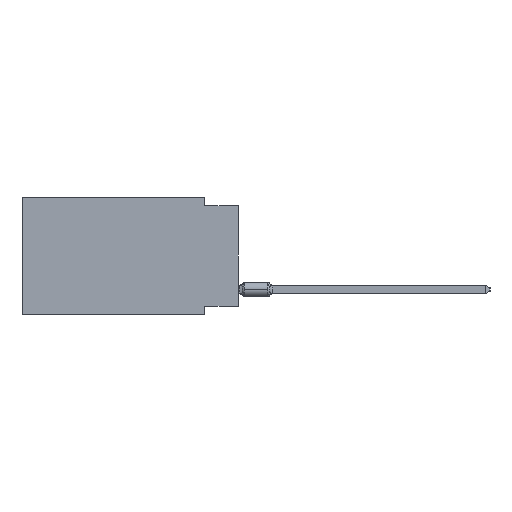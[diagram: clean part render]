
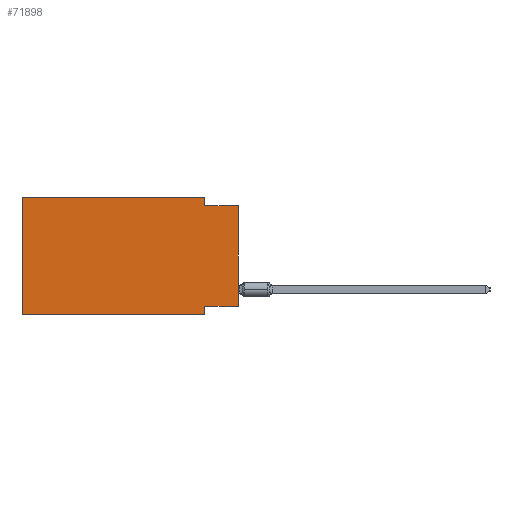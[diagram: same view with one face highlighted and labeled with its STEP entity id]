
A CAD part, left-side view. The second image highlights one B-rep face of the part: STEP entity #71898.
In plain terms, the highlighted planar face has unit normal (-1, 0, 0).
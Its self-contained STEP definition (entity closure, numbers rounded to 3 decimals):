
#1831 = VECTOR ( 'NONE', #77234, 1000. ) ;
#3227 = ORIENTED_EDGE ( 'NONE', *, *, #85287, .T. ) ;
#4537 = CARTESIAN_POINT ( 'NONE',  ( 0., 0., -0.635 ) ) ;
#5305 = LINE ( 'NONE', #25249, #21203 ) ;
#6075 = VECTOR ( 'NONE', #18033, 1000. ) ;
#7210 = ORIENTED_EDGE ( 'NONE', *, *, #81628, .F. ) ;
#7359 = ORIENTED_EDGE ( 'NONE', *, *, #38900, .F. ) ;
#11522 = DIRECTION ( 'NONE',  ( 0., 0., 1. ) ) ;
#11753 = ORIENTED_EDGE ( 'NONE', *, *, #20453, .F. ) ;
#14255 = CARTESIAN_POINT ( 'NONE',  ( 0., 0., -8.255 ) ) ;
#15845 = DIRECTION ( 'NONE',  ( 0., 0., 1. ) ) ;
#16922 = PLANE ( 'NONE',  #84972 ) ;
#17297 = LINE ( 'NONE', #45602, #70333 ) ;
#18033 = DIRECTION ( 'NONE',  ( 0., -1., 0. ) ) ;
#20453 = EDGE_CURVE ( 'NONE', #43171, #83432, #17297, .T. ) ;
#20618 = LINE ( 'NONE', #71031, #1831 ) ;
#21145 = CARTESIAN_POINT ( 'NONE',  ( 0., 16.383, -8.89 ) ) ;
#21203 = VECTOR ( 'NONE', #11522, 1000. ) ;
#21328 = VERTEX_POINT ( 'NONE', #14255 ) ;
#23291 = LINE ( 'NONE', #68447, #70757 ) ;
#25249 = CARTESIAN_POINT ( 'NONE',  ( 0., 0., 0. ) ) ;
#25520 = ORIENTED_EDGE ( 'NONE', *, *, #26877, .T. ) ;
#26877 = EDGE_CURVE ( 'NONE', #47099, #83432, #78660, .T. ) ;
#27640 = DIRECTION ( 'NONE',  ( 0., 0., -1. ) ) ;
#29930 = DIRECTION ( 'NONE',  ( 0., 1., 0. ) ) ;
#32141 = CARTESIAN_POINT ( 'NONE',  ( 0., 2.54, -8.255 ) ) ;
#35023 = VERTEX_POINT ( 'NONE', #84285 ) ;
#35749 = LINE ( 'NONE', #62773, #77316 ) ;
#38900 = EDGE_CURVE ( 'NONE', #47099, #35023, #35749, .T. ) ;
#39624 = LINE ( 'NONE', #46261, #44799 ) ;
#39806 = EDGE_LOOP ( 'NONE', ( #3227, #79651, #7210, #78888, #7359, #25520, #11753, #62754 ) ) ;
#39841 = LINE ( 'NONE', #53557, #54828 ) ;
#42591 = DIRECTION ( 'NONE',  ( 0., 0., -1. ) ) ;
#43171 = VERTEX_POINT ( 'NONE', #32141 ) ;
#44799 = VECTOR ( 'NONE', #27640, 1000. ) ;
#45602 = CARTESIAN_POINT ( 'NONE',  ( 0., 2.54, -8.89 ) ) ;
#46261 = CARTESIAN_POINT ( 'NONE',  ( 0., 2.54, 0. ) ) ;
#47099 = VERTEX_POINT ( 'NONE', #21145 ) ;
#47424 = VERTEX_POINT ( 'NONE', #52097 ) ;
#52097 = CARTESIAN_POINT ( 'NONE',  ( 0., 2.54, 0. ) ) ;
#53557 = CARTESIAN_POINT ( 'NONE',  ( 0., 0., -0.635 ) ) ;
#54108 = VERTEX_POINT ( 'NONE', #56656 ) ;
#54828 = VECTOR ( 'NONE', #81847, 1000. ) ;
#56656 = CARTESIAN_POINT ( 'NONE',  ( 0., 2.54, -0.635 ) ) ;
#61626 = CARTESIAN_POINT ( 'NONE',  ( 0., 2.54, -8.89 ) ) ;
#62754 = ORIENTED_EDGE ( 'NONE', *, *, #85864, .F. ) ;
#62773 = CARTESIAN_POINT ( 'NONE',  ( 0., 16.383, 0. ) ) ;
#68447 = CARTESIAN_POINT ( 'NONE',  ( 0., 0., -8.255 ) ) ;
#68719 = DIRECTION ( 'NONE',  ( 1., 0., 0. ) ) ;
#70333 = VECTOR ( 'NONE', #77931, 1000. ) ;
#70757 = VECTOR ( 'NONE', #29930, 1000. ) ;
#71031 = CARTESIAN_POINT ( 'NONE',  ( 0., 16.383, 0. ) ) ;
#71898 = ADVANCED_FACE ( 'NONE', ( #77120 ), #16922, .F. ) ;
#73950 = EDGE_CURVE ( 'NONE', #35023, #47424, #20618, .T. ) ;
#77120 = FACE_OUTER_BOUND ( 'NONE', #39806, .T. ) ;
#77234 = DIRECTION ( 'NONE',  ( 0., -1., 0. ) ) ;
#77316 = VECTOR ( 'NONE', #15845, 1000. ) ;
#77931 = DIRECTION ( 'NONE',  ( 0., 0., -1. ) ) ;
#78660 = LINE ( 'NONE', #85743, #6075 ) ;
#78888 = ORIENTED_EDGE ( 'NONE', *, *, #73950, .F. ) ;
#79546 = VERTEX_POINT ( 'NONE', #4537 ) ;
#79651 = ORIENTED_EDGE ( 'NONE', *, *, #82527, .F. ) ;
#81628 = EDGE_CURVE ( 'NONE', #47424, #54108, #39624, .T. ) ;
#81847 = DIRECTION ( 'NONE',  ( 0., -1., 0. ) ) ;
#82527 = EDGE_CURVE ( 'NONE', #54108, #79546, #39841, .T. ) ;
#83300 = CARTESIAN_POINT ( 'NONE',  ( 0., 16.383, 0. ) ) ;
#83432 = VERTEX_POINT ( 'NONE', #61626 ) ;
#84285 = CARTESIAN_POINT ( 'NONE',  ( 0., 16.383, 0. ) ) ;
#84972 = AXIS2_PLACEMENT_3D ( 'NONE', #83300, #68719, #42591 ) ;
#85287 = EDGE_CURVE ( 'NONE', #21328, #79546, #5305, .T. ) ;
#85743 = CARTESIAN_POINT ( 'NONE',  ( 0., 16.383, -8.89 ) ) ;
#85864 = EDGE_CURVE ( 'NONE', #21328, #43171, #23291, .T. ) ;
